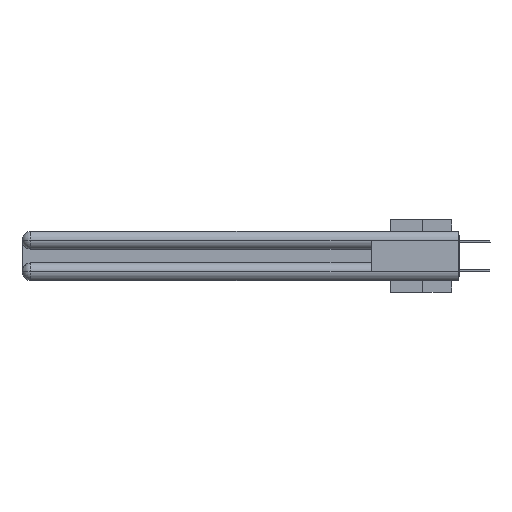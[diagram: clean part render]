
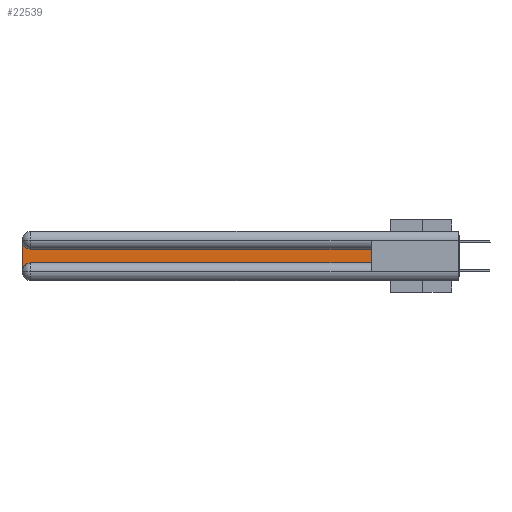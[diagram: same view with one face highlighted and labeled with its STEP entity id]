
A CAD part, left-side view. The second image highlights one B-rep face of the part: STEP entity #22539.
In plain terms, the highlighted planar face has unit normal (-1, 0, 0).
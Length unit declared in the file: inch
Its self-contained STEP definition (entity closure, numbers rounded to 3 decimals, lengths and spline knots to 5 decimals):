
#353 = EDGE_CURVE ( 'NONE', #24159, #20356, #2037, .T. ) ;
#929 = DIRECTION ( 'NONE',  ( 0., 0., -1. ) ) ;
#1063 = LINE ( 'NONE', #3569, #31648 ) ;
#1145 = VECTOR ( 'NONE', #1618, 39.37008 ) ;
#1231 = CARTESIAN_POINT ( 'NONE',  ( 0.075, 2.94, -0.2775 ) ) ;
#1618 = DIRECTION ( 'NONE',  ( 0., 0., -1. ) ) ;
#2037 = CIRCLE ( 'NONE', #27028, 0.06 ) ;
#3569 = CARTESIAN_POINT ( 'NONE',  ( 0.075, 0.6, -0.2175 ) ) ;
#3611 = CARTESIAN_POINT ( 'NONE',  ( 0.075, 0.6, -0.1225 ) ) ;
#3939 = DIRECTION ( 'NONE',  ( 0., 0., -1. ) ) ;
#4270 = EDGE_CURVE ( 'NONE', #11738, #13401, #12811, .T. ) ;
#4646 = EDGE_LOOP ( 'NONE', ( #11204, #12882, #22113, #18528, #6377, #8381 ) ) ;
#5064 = VERTEX_POINT ( 'NONE', #3611 ) ;
#5659 = VECTOR ( 'NONE', #11824, 39.37008 ) ;
#5827 = PLANE ( 'NONE',  #27949 ) ;
#6377 = ORIENTED_EDGE ( 'NONE', *, *, #15485, .T. ) ;
#6505 = AXIS2_PLACEMENT_3D ( 'NONE', #16988, #27839, #929 ) ;
#8381 = ORIENTED_EDGE ( 'NONE', *, *, #32390, .T. ) ;
#8432 = CARTESIAN_POINT ( 'NONE',  ( 0.075, 0.6, -0.1225 ) ) ;
#9097 = CARTESIAN_POINT ( 'NONE',  ( 0.075, 0.6, -0.2175 ) ) ;
#10024 = LINE ( 'NONE', #8432, #23381 ) ;
#11145 = DIRECTION ( 'NONE',  ( 0., 0., -1. ) ) ;
#11204 = ORIENTED_EDGE ( 'NONE', *, *, #26820, .T. ) ;
#11738 = VERTEX_POINT ( 'NONE', #30760 ) ;
#11824 = DIRECTION ( 'NONE',  ( 0., -1., 0. ) ) ;
#12270 = VERTEX_POINT ( 'NONE', #24309 ) ;
#12811 = CIRCLE ( 'NONE', #6505, 0.06 ) ;
#12816 = LINE ( 'NONE', #9097, #5659 ) ;
#12882 = ORIENTED_EDGE ( 'NONE', *, *, #4270, .T. ) ;
#13142 = EDGE_CURVE ( 'NONE', #13401, #24159, #17155, .T. ) ;
#13401 = VERTEX_POINT ( 'NONE', #32687 ) ;
#15485 = EDGE_CURVE ( 'NONE', #20356, #12270, #12816, .T. ) ;
#16988 = CARTESIAN_POINT ( 'NONE',  ( 0.075, 2.94, -0.0625 ) ) ;
#17155 = LINE ( 'NONE', #23032, #1145 ) ;
#17779 = DIRECTION ( 'NONE',  ( 1., 0., 0. ) ) ;
#18528 = ORIENTED_EDGE ( 'NONE', *, *, #353, .T. ) ;
#19009 = DIRECTION ( 'NONE',  ( 0., 1., 0. ) ) ;
#20356 = VERTEX_POINT ( 'NONE', #28927 ) ;
#21885 = DIRECTION ( 'NONE',  ( 1., 0., 0. ) ) ;
#22000 = CARTESIAN_POINT ( 'NONE',  ( 0.075, 3., -0.1225 ) ) ;
#22113 = ORIENTED_EDGE ( 'NONE', *, *, #13142, .T. ) ;
#22539 = ADVANCED_FACE ( 'NONE', ( #31566 ), #5827, .F. ) ;
#22947 = CARTESIAN_POINT ( 'NONE',  ( 0.075, 3., -0.2775 ) ) ;
#23032 = CARTESIAN_POINT ( 'NONE',  ( 0.075, 3., -0.2175 ) ) ;
#23381 = VECTOR ( 'NONE', #19009, 39.37008 ) ;
#24159 = VERTEX_POINT ( 'NONE', #22947 ) ;
#24309 = CARTESIAN_POINT ( 'NONE',  ( 0.075, 0.6, -0.2175 ) ) ;
#26820 = EDGE_CURVE ( 'NONE', #5064, #11738, #10024, .T. ) ;
#27028 = AXIS2_PLACEMENT_3D ( 'NONE', #1231, #17779, #3939 ) ;
#27839 = DIRECTION ( 'NONE',  ( 1., 0., 0. ) ) ;
#27949 = AXIS2_PLACEMENT_3D ( 'NONE', #22000, #21885, #11145 ) ;
#28927 = CARTESIAN_POINT ( 'NONE',  ( 0.075, 2.94, -0.2175 ) ) ;
#30664 = DIRECTION ( 'NONE',  ( 0., 0., 1. ) ) ;
#30760 = CARTESIAN_POINT ( 'NONE',  ( 0.075, 2.94, -0.1225 ) ) ;
#31566 = FACE_OUTER_BOUND ( 'NONE', #4646, .T. ) ;
#31648 = VECTOR ( 'NONE', #30664, 39.37008 ) ;
#32390 = EDGE_CURVE ( 'NONE', #12270, #5064, #1063, .T. ) ;
#32687 = CARTESIAN_POINT ( 'NONE',  ( 0.075, 3., -0.0625 ) ) ;
